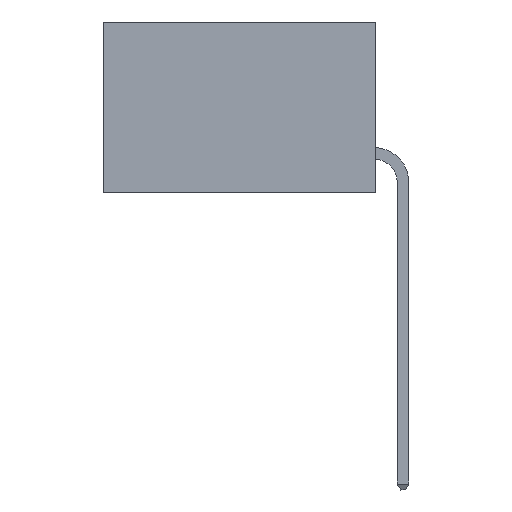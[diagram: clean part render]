
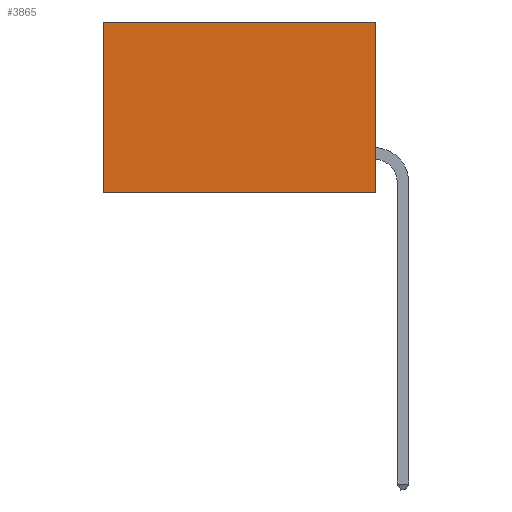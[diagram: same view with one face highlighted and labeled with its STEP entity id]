
A CAD part, left-side view. The second image highlights one B-rep face of the part: STEP entity #3865.
In plain terms, the highlighted planar face has unit normal (-1, 0, 0).
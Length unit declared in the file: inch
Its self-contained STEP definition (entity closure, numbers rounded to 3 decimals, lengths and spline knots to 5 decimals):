
#448 = ORIENTED_EDGE ( 'NONE', *, *, #3373, .T. ) ;
#561 = VECTOR ( 'NONE', #2580, 39.37008 ) ;
#848 = LINE ( 'NONE', #4688, #4249 ) ;
#871 = DIRECTION ( 'NONE',  ( 0., 1., 0. ) ) ;
#1280 = EDGE_CURVE ( 'NONE', #4227, #2534, #6412, .T. ) ;
#1938 = CARTESIAN_POINT ( 'NONE',  ( 0.277, 0.59, -0.37 ) ) ;
#1953 = CARTESIAN_POINT ( 'NONE',  ( 0.277, 0., -0.37 ) ) ;
#1990 = PLANE ( 'NONE',  #5490 ) ;
#2149 = CARTESIAN_POINT ( 'NONE',  ( 0.277, 0.59, -0.37 ) ) ;
#2418 = ORIENTED_EDGE ( 'NONE', *, *, #3181, .F. ) ;
#2534 = VERTEX_POINT ( 'NONE', #1938 ) ;
#2580 = DIRECTION ( 'NONE',  ( 0., 0., -1. ) ) ;
#2632 = VERTEX_POINT ( 'NONE', #4084 ) ;
#2707 = ORIENTED_EDGE ( 'NONE', *, *, #1280, .T. ) ;
#2895 = CARTESIAN_POINT ( 'NONE',  ( 0.277, 0., -0.37 ) ) ;
#3181 = EDGE_CURVE ( 'NONE', #2632, #3519, #7356, .T. ) ;
#3214 = VECTOR ( 'NONE', #6625, 39.37008 ) ;
#3281 = DIRECTION ( 'NONE',  ( 1., 0., 0. ) ) ;
#3373 = EDGE_CURVE ( 'NONE', #2632, #4227, #848, .T. ) ;
#3519 = VERTEX_POINT ( 'NONE', #2895 ) ;
#3610 = VECTOR ( 'NONE', #3699, 39.37008 ) ;
#3699 = DIRECTION ( 'NONE',  ( 0., 1., 0. ) ) ;
#3733 = CARTESIAN_POINT ( 'NONE',  ( 0.277, 0., -0.37 ) ) ;
#3865 = ADVANCED_FACE ( 'NONE', ( #3918 ), #1990, .F. ) ;
#3918 = FACE_OUTER_BOUND ( 'NONE', #6663, .T. ) ;
#4084 = CARTESIAN_POINT ( 'NONE',  ( 0.277, 0., 0. ) ) ;
#4227 = VERTEX_POINT ( 'NONE', #5297 ) ;
#4249 = VECTOR ( 'NONE', #871, 39.37008 ) ;
#4568 = EDGE_CURVE ( 'NONE', #3519, #2534, #7006, .T. ) ;
#4688 = CARTESIAN_POINT ( 'NONE',  ( 0.277, 0., 0. ) ) ;
#5297 = CARTESIAN_POINT ( 'NONE',  ( 0.277, 0.59, 0. ) ) ;
#5490 = AXIS2_PLACEMENT_3D ( 'NONE', #7116, #3281, #7764 ) ;
#6325 = ORIENTED_EDGE ( 'NONE', *, *, #4568, .F. ) ;
#6412 = LINE ( 'NONE', #2149, #3214 ) ;
#6625 = DIRECTION ( 'NONE',  ( 0., 0., -1. ) ) ;
#6663 = EDGE_LOOP ( 'NONE', ( #2707, #6325, #2418, #448 ) ) ;
#7006 = LINE ( 'NONE', #3733, #3610 ) ;
#7116 = CARTESIAN_POINT ( 'NONE',  ( 0.277, 0., -0.37 ) ) ;
#7356 = LINE ( 'NONE', #1953, #561 ) ;
#7764 = DIRECTION ( 'NONE',  ( 0., 0., -1. ) ) ;
